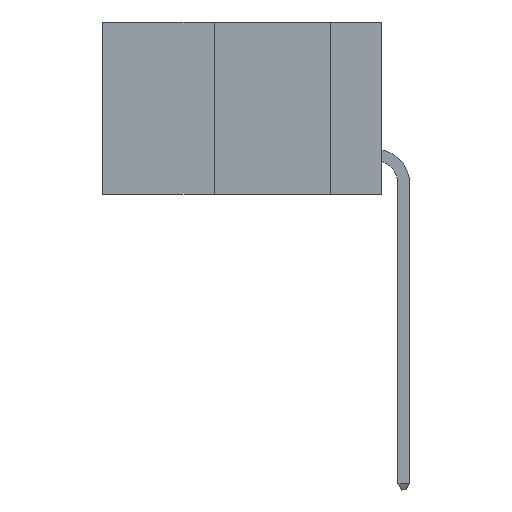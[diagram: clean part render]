
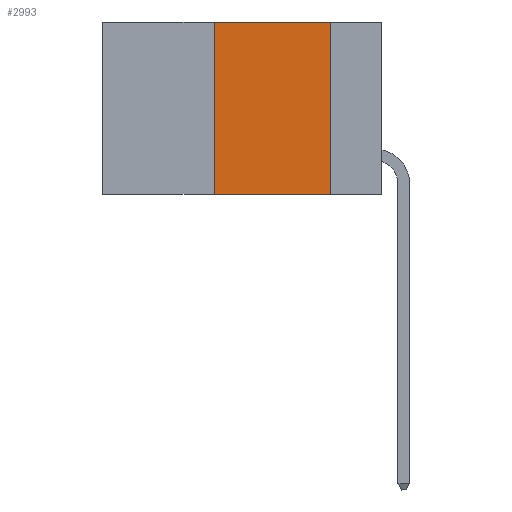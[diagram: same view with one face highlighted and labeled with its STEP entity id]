
A CAD part, left-side view. The second image highlights one B-rep face of the part: STEP entity #2993.
In plain terms, the highlighted planar face has unit normal (-1, 0, 0).
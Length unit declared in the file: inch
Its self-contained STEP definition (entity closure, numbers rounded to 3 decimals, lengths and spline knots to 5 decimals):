
#20 = VECTOR ( 'NONE', #13774, 39.37008 ) ;
#671 = DIRECTION ( 'NONE',  ( 0., 0., -1. ) ) ;
#1271 = DIRECTION ( 'NONE',  ( 0., -1., 0. ) ) ;
#1776 = CARTESIAN_POINT ( 'NONE',  ( 0., 0.11, 0. ) ) ;
#2057 = DIRECTION ( 'NONE',  ( 0., -1., 0. ) ) ;
#2656 = ORIENTED_EDGE ( 'NONE', *, *, #6277, .F. ) ;
#2704 = CARTESIAN_POINT ( 'NONE',  ( 0., 0.6, 0. ) ) ;
#2893 = FACE_OUTER_BOUND ( 'NONE', #12920, .T. ) ;
#2993 = ADVANCED_FACE ( 'NONE', ( #2893 ), #13858, .F. ) ;
#4221 = VERTEX_POINT ( 'NONE', #15440 ) ;
#5260 = CARTESIAN_POINT ( 'NONE',  ( 0., 0.36, -0.37 ) ) ;
#5969 = CARTESIAN_POINT ( 'NONE',  ( 0., 0.11, 0. ) ) ;
#6277 = EDGE_CURVE ( 'NONE', #12443, #14391, #8189, .T. ) ;
#6929 = CARTESIAN_POINT ( 'NONE',  ( 0., 0.6, -0.37 ) ) ;
#6991 = VECTOR ( 'NONE', #2057, 39.37008 ) ;
#7101 = CARTESIAN_POINT ( 'NONE',  ( 0., 0.11, -0.37 ) ) ;
#7515 = ORIENTED_EDGE ( 'NONE', *, *, #14848, .F. ) ;
#7931 = CARTESIAN_POINT ( 'NONE',  ( 0., 0.36, 0. ) ) ;
#8189 = LINE ( 'NONE', #1776, #20 ) ;
#8332 = VECTOR ( 'NONE', #15284, 39.37008 ) ;
#8769 = EDGE_CURVE ( 'NONE', #11416, #14391, #10203, .T. ) ;
#8962 = CARTESIAN_POINT ( 'NONE',  ( 0., 0.6, 0. ) ) ;
#10203 = LINE ( 'NONE', #6929, #6991 ) ;
#11416 = VERTEX_POINT ( 'NONE', #5260 ) ;
#12021 = EDGE_CURVE ( 'NONE', #4221, #12443, #14257, .T. ) ;
#12189 = ORIENTED_EDGE ( 'NONE', *, *, #8769, .T. ) ;
#12443 = VERTEX_POINT ( 'NONE', #5969 ) ;
#12920 = EDGE_LOOP ( 'NONE', ( #2656, #13265, #7515, #12189 ) ) ;
#13212 = AXIS2_PLACEMENT_3D ( 'NONE', #8962, #15199, #671 ) ;
#13265 = ORIENTED_EDGE ( 'NONE', *, *, #12021, .F. ) ;
#13774 = DIRECTION ( 'NONE',  ( 0., 0., -1. ) ) ;
#13858 = PLANE ( 'NONE',  #13212 ) ;
#14257 = LINE ( 'NONE', #2704, #15216 ) ;
#14391 = VERTEX_POINT ( 'NONE', #7101 ) ;
#14563 = LINE ( 'NONE', #7931, #8332 ) ;
#14848 = EDGE_CURVE ( 'NONE', #11416, #4221, #14563, .T. ) ;
#15199 = DIRECTION ( 'NONE',  ( 1., 0., 0. ) ) ;
#15216 = VECTOR ( 'NONE', #1271, 39.37008 ) ;
#15284 = DIRECTION ( 'NONE',  ( 0., 0., 1. ) ) ;
#15440 = CARTESIAN_POINT ( 'NONE',  ( 0., 0.36, 0. ) ) ;
